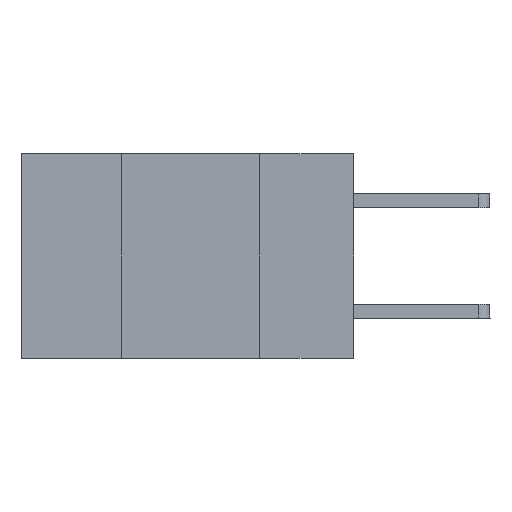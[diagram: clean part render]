
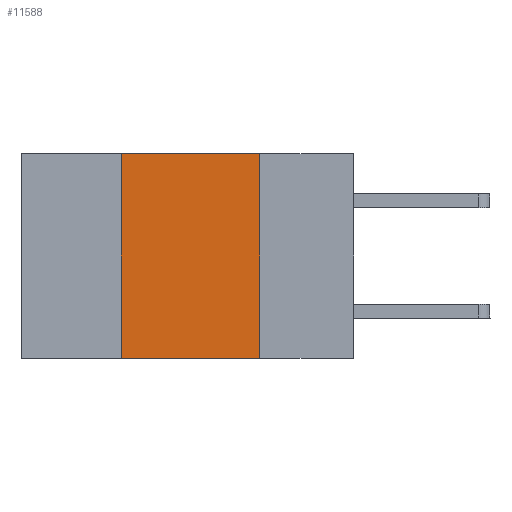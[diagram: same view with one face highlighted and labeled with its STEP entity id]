
A CAD part, left-side view. The second image highlights one B-rep face of the part: STEP entity #11588.
In plain terms, the highlighted planar face has unit normal (-1, 0, 0).
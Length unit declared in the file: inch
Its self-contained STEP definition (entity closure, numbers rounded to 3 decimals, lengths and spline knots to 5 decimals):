
#336 = CARTESIAN_POINT ( 'NONE',  ( 0., 0.6, 0. ) ) ;
#1058 = DIRECTION ( 'NONE',  ( 0., 0., -1. ) ) ;
#1678 = VECTOR ( 'NONE', #9980, 39.37008 ) ;
#1741 = DIRECTION ( 'NONE',  ( 0., 0., 1. ) ) ;
#1993 = ORIENTED_EDGE ( 'NONE', *, *, #14000, .F. ) ;
#2342 = DIRECTION ( 'NONE',  ( 1., 0., 0. ) ) ;
#2466 = CARTESIAN_POINT ( 'NONE',  ( 0., 0.42, 0. ) ) ;
#2510 = CARTESIAN_POINT ( 'NONE',  ( 0., 0.17, -0.37 ) ) ;
#2605 = EDGE_CURVE ( 'NONE', #6669, #13097, #12924, .T. ) ;
#3256 = VECTOR ( 'NONE', #1741, 39.37008 ) ;
#3425 = ORIENTED_EDGE ( 'NONE', *, *, #14394, .T. ) ;
#3499 = AXIS2_PLACEMENT_3D ( 'NONE', #11033, #2342, #1058 ) ;
#3739 = CARTESIAN_POINT ( 'NONE',  ( 0., 0.17, 0. ) ) ;
#4144 = LINE ( 'NONE', #336, #1678 ) ;
#4616 = FACE_OUTER_BOUND ( 'NONE', #14252, .T. ) ;
#5470 = DIRECTION ( 'NONE',  ( 0., 0., -1. ) ) ;
#5708 = CARTESIAN_POINT ( 'NONE',  ( 0., 0.17, 0. ) ) ;
#5757 = PLANE ( 'NONE',  #3499 ) ;
#5848 = CARTESIAN_POINT ( 'NONE',  ( 0., 0.6, -0.37 ) ) ;
#6080 = VERTEX_POINT ( 'NONE', #6887 ) ;
#6669 = VERTEX_POINT ( 'NONE', #3739 ) ;
#6887 = CARTESIAN_POINT ( 'NONE',  ( 0., 0.42, -0.37 ) ) ;
#6902 = EDGE_CURVE ( 'NONE', #8967, #6669, #4144, .T. ) ;
#7497 = ORIENTED_EDGE ( 'NONE', *, *, #2605, .F. ) ;
#8967 = VERTEX_POINT ( 'NONE', #10106 ) ;
#9980 = DIRECTION ( 'NONE',  ( 0., -1., 0. ) ) ;
#10106 = CARTESIAN_POINT ( 'NONE',  ( 0., 0.42, 0. ) ) ;
#10322 = DIRECTION ( 'NONE',  ( 0., -1., 0. ) ) ;
#11033 = CARTESIAN_POINT ( 'NONE',  ( 0., 0.6, 0. ) ) ;
#11588 = ADVANCED_FACE ( 'NONE', ( #4616 ), #5757, .F. ) ;
#12924 = LINE ( 'NONE', #5708, #15491 ) ;
#13097 = VERTEX_POINT ( 'NONE', #2510 ) ;
#13573 = LINE ( 'NONE', #2466, #3256 ) ;
#14000 = EDGE_CURVE ( 'NONE', #6080, #8967, #13573, .T. ) ;
#14252 = EDGE_LOOP ( 'NONE', ( #7497, #15312, #1993, #3425 ) ) ;
#14394 = EDGE_CURVE ( 'NONE', #6080, #13097, #15735, .T. ) ;
#15312 = ORIENTED_EDGE ( 'NONE', *, *, #6902, .F. ) ;
#15446 = VECTOR ( 'NONE', #10322, 39.37008 ) ;
#15491 = VECTOR ( 'NONE', #5470, 39.37008 ) ;
#15735 = LINE ( 'NONE', #5848, #15446 ) ;
